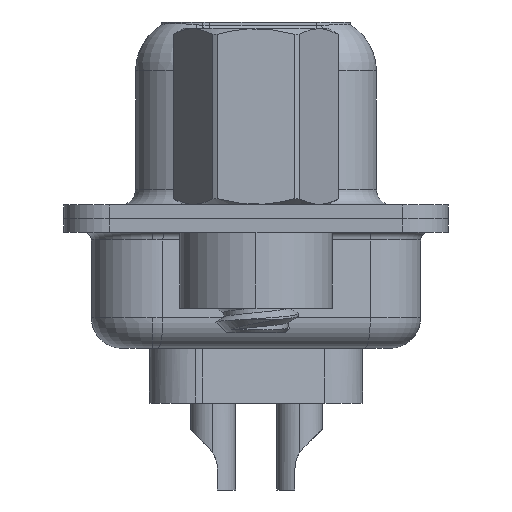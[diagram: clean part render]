
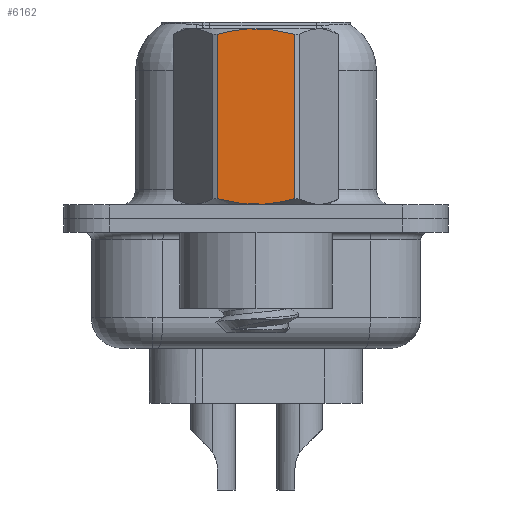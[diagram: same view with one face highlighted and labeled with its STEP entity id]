
A CAD part, left-side view. The second image highlights one B-rep face of the part: STEP entity #6162.
In plain terms, the highlighted planar face has unit normal (-1, 0, 0).
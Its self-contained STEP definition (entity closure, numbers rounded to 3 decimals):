
#632 = B_SPLINE_CURVE_WITH_KNOTS ( 'NONE', 3,
 ( #18849, #13277, #7864, #11586, #7504, #2273, #22365, #9678, #13156, #20443 ),
 .UNSPECIFIED., .F., .F.,
 ( 4, 2, 2, 2, 4 ),
 ( 0.001, 0.002, 0.002, 0.003, 0.004 ),
 .UNSPECIFIED. ) ;
#1323 = ORIENTED_EDGE ( 'NONE', *, *, #23347, .T. ) ;
#1928 = VECTOR ( 'NONE', #2684, 1000. ) ;
#2273 = CARTESIAN_POINT ( 'NONE',  ( -2.381, 0.215, 6.232 ) ) ;
#2684 = DIRECTION ( 'NONE',  ( 0., 0., -1. ) ) ;
#2808 = CARTESIAN_POINT ( 'NONE',  ( -2.381, -0.432, 0.485 ) ) ;
#3033 = CARTESIAN_POINT ( 'NONE',  ( -2.381, 1.273, 3.792 ) ) ;
#3215 = AXIS2_PLACEMENT_3D ( 'NONE', #23365, #19494, #23482 ) ;
#3536 = VERTEX_POINT ( 'NONE', #5688 ) ;
#3668 = B_SPLINE_CURVE_WITH_KNOTS ( 'NONE', 3,
 ( #10202, #4642, #15533, #15766, #11995, #19381, #2808, #23139, #12116, #19504 ),
 .UNSPECIFIED., .F., .F.,
 ( 4, 2, 2, 2, 4 ),
 ( 0.003, 0.003, 0.004, 0.004, 0.005 ),
 .UNSPECIFIED. ) ;
#4642 = CARTESIAN_POINT ( 'NONE',  ( -2.381, 1.065, 0.596 ) ) ;
#5688 = CARTESIAN_POINT ( 'NONE',  ( -2.381, -1.273, 0.652 ) ) ;
#5746 = CARTESIAN_POINT ( 'NONE',  ( -2.381, 1.273, 0.652 ) ) ;
#5927 = EDGE_LOOP ( 'NONE', ( #20502, #16560, #6973, #1323 ) ) ;
#6162 = ADVANCED_FACE ( 'NONE', ( #23129 ), #15999, .T. ) ;
#6973 = ORIENTED_EDGE ( 'NONE', *, *, #12665, .T. ) ;
#7504 = CARTESIAN_POINT ( 'NONE',  ( -2.381, -0.215, 6.232 ) ) ;
#7864 = CARTESIAN_POINT ( 'NONE',  ( -2.381, -0.858, 6.15 ) ) ;
#8682 = LINE ( 'NONE', #16039, #9324 ) ;
#8841 = VERTEX_POINT ( 'NONE', #5746 ) ;
#8980 = EDGE_CURVE ( 'NONE', #8841, #3536, #3668, .T. ) ;
#9324 = VECTOR ( 'NONE', #23401, 1000. ) ;
#9678 = CARTESIAN_POINT ( 'NONE',  ( -2.381, 0.853, 6.151 ) ) ;
#10202 = CARTESIAN_POINT ( 'NONE',  ( -2.381, 1.273, 0.652 ) ) ;
#11288 = VERTEX_POINT ( 'NONE', #11813 ) ;
#11586 = CARTESIAN_POINT ( 'NONE',  ( -2.381, -0.432, 6.215 ) ) ;
#11813 = CARTESIAN_POINT ( 'NONE',  ( -2.381, 1.273, 6.048 ) ) ;
#11995 = CARTESIAN_POINT ( 'NONE',  ( -2.381, 0.215, 0.468 ) ) ;
#12111 = LINE ( 'NONE', #3033, #1928 ) ;
#12116 = CARTESIAN_POINT ( 'NONE',  ( -2.381, -1.066, 0.596 ) ) ;
#12665 = EDGE_CURVE ( 'NONE', #23391, #11288, #632, .T. ) ;
#13156 = CARTESIAN_POINT ( 'NONE',  ( -2.381, 1.065, 6.104 ) ) ;
#13277 = CARTESIAN_POINT ( 'NONE',  ( -2.381, -1.066, 6.104 ) ) ;
#14092 = EDGE_CURVE ( 'NONE', #3536, #23391, #8682, .T. ) ;
#15533 = CARTESIAN_POINT ( 'NONE',  ( -2.381, 0.853, 0.549 ) ) ;
#15766 = CARTESIAN_POINT ( 'NONE',  ( -2.381, 0.428, 0.485 ) ) ;
#15884 = CARTESIAN_POINT ( 'NONE',  ( -2.381, -1.273, 6.048 ) ) ;
#15999 = PLANE ( 'NONE',  #3215 ) ;
#16039 = CARTESIAN_POINT ( 'NONE',  ( -2.381, -1.273, 3.792 ) ) ;
#16560 = ORIENTED_EDGE ( 'NONE', *, *, #14092, .T. ) ;
#18849 = CARTESIAN_POINT ( 'NONE',  ( -2.381, -1.273, 6.048 ) ) ;
#19381 = CARTESIAN_POINT ( 'NONE',  ( -2.381, -0.215, 0.468 ) ) ;
#19494 = DIRECTION ( 'NONE',  ( -1., 0., 0. ) ) ;
#19504 = CARTESIAN_POINT ( 'NONE',  ( -2.381, -1.273, 0.652 ) ) ;
#20443 = CARTESIAN_POINT ( 'NONE',  ( -2.381, 1.273, 6.048 ) ) ;
#20502 = ORIENTED_EDGE ( 'NONE', *, *, #8980, .T. ) ;
#22365 = CARTESIAN_POINT ( 'NONE',  ( -2.381, 0.428, 6.215 ) ) ;
#23129 = FACE_OUTER_BOUND ( 'NONE', #5927, .T. ) ;
#23139 = CARTESIAN_POINT ( 'NONE',  ( -2.381, -0.858, 0.55 ) ) ;
#23347 = EDGE_CURVE ( 'NONE', #11288, #8841, #12111, .T. ) ;
#23365 = CARTESIAN_POINT ( 'NONE',  ( -2.381, 1.375, -3.75 ) ) ;
#23391 = VERTEX_POINT ( 'NONE', #15884 ) ;
#23401 = DIRECTION ( 'NONE',  ( 0., 0., 1. ) ) ;
#23482 = DIRECTION ( 'NONE',  ( 0., -1., 0. ) ) ;
